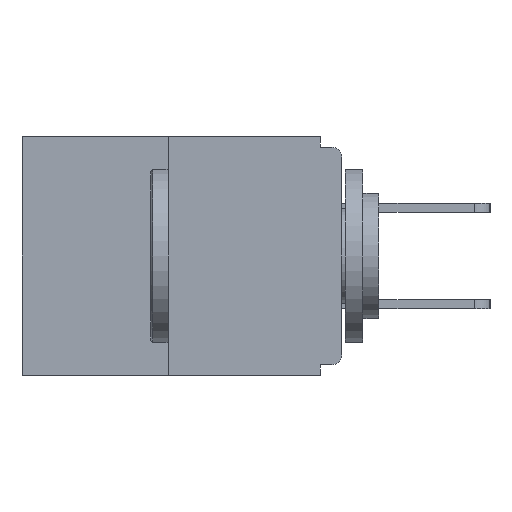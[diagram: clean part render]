
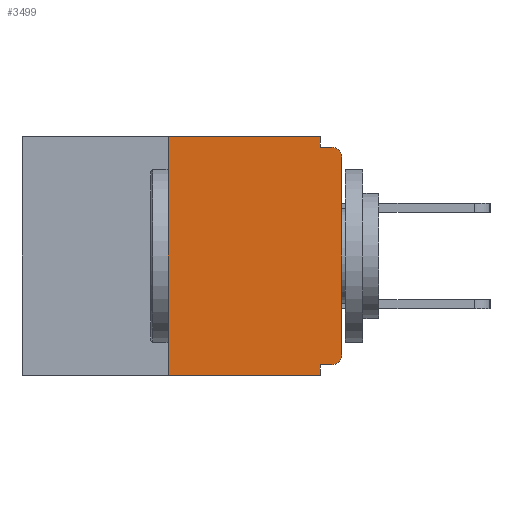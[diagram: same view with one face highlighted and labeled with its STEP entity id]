
A CAD part, left-side view. The second image highlights one B-rep face of the part: STEP entity #3499.
In plain terms, the highlighted planar face has unit normal (-1, 0, 0).
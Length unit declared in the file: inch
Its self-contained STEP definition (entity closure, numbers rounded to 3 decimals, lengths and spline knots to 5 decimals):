
#41 = CARTESIAN_POINT ( 'NONE',  ( 0., 0.015, -0.015 ) ) ;
#445 = CARTESIAN_POINT ( 'NONE',  ( 0., 0.015, -0.03 ) ) ;
#483 = DIRECTION ( 'NONE',  ( 1., 0., 0. ) ) ;
#566 = PLANE ( 'NONE',  #16511 ) ;
#655 = CARTESIAN_POINT ( 'NONE',  ( 0., 0.015, -0.328 ) ) ;
#1025 = CARTESIAN_POINT ( 'NONE',  ( 0., 0.031, 0. ) ) ;
#1550 = VERTEX_POINT ( 'NONE', #13295 ) ;
#2304 = VERTEX_POINT ( 'NONE', #9334 ) ;
#2338 = VERTEX_POINT ( 'NONE', #655 ) ;
#2637 = VERTEX_POINT ( 'NONE', #28172 ) ;
#2711 = DIRECTION ( 'NONE',  ( -1., 0., 0. ) ) ;
#2716 = DIRECTION ( 'NONE',  ( 0., -1., 0. ) ) ;
#3070 = VECTOR ( 'NONE', #3271, 39.37008 ) ;
#3271 = DIRECTION ( 'NONE',  ( 0., -1., 0. ) ) ;
#3492 = EDGE_CURVE ( 'NONE', #14573, #27161, #8986, .T. ) ;
#3499 = ADVANCED_FACE ( 'NONE', ( #24289 ), #566, .F. ) ;
#3878 = ORIENTED_EDGE ( 'NONE', *, *, #14083, .F. ) ;
#4466 = VERTEX_POINT ( 'NONE', #18391 ) ;
#4516 = VERTEX_POINT ( 'NONE', #1025 ) ;
#4928 = AXIS2_PLACEMENT_3D ( 'NONE', #20759, #5665, #27473 ) ;
#4995 = DIRECTION ( 'NONE',  ( 0., 0., -1. ) ) ;
#5268 = EDGE_CURVE ( 'NONE', #14573, #2637, #14663, .T. ) ;
#5332 = CARTESIAN_POINT ( 'NONE',  ( 0., 0.46, -0.343 ) ) ;
#5359 = EDGE_LOOP ( 'NONE', ( #6457, #19528, #24712, #18139, #14676, #10638, #19654, #18191, #3878, #10614 ) ) ;
#5665 = DIRECTION ( 'NONE',  ( -1., 0., 0. ) ) ;
#6179 = DIRECTION ( 'NONE',  ( 0., 0., -1. ) ) ;
#6457 = ORIENTED_EDGE ( 'NONE', *, *, #12551, .F. ) ;
#6842 = CARTESIAN_POINT ( 'NONE',  ( 0., 0.031, -0.015 ) ) ;
#6968 = CARTESIAN_POINT ( 'NONE',  ( 0., 0.46, 0. ) ) ;
#7500 = LINE ( 'NONE', #14070, #3070 ) ;
#8016 = VECTOR ( 'NONE', #6179, 39.37008 ) ;
#8986 = LINE ( 'NONE', #22368, #21553 ) ;
#9126 = CARTESIAN_POINT ( 'NONE',  ( 0., 0.25, 0. ) ) ;
#9263 = VERTEX_POINT ( 'NONE', #41 ) ;
#9334 = CARTESIAN_POINT ( 'NONE',  ( 0., 0., -0.313 ) ) ;
#9336 = DIRECTION ( 'NONE',  ( 0., 0., -1. ) ) ;
#9657 = EDGE_CURVE ( 'NONE', #4516, #13980, #14191, .T. ) ;
#9791 = VECTOR ( 'NONE', #2716, 39.37008 ) ;
#10184 = DIRECTION ( 'NONE',  ( 0., 0., -1. ) ) ;
#10614 = ORIENTED_EDGE ( 'NONE', *, *, #9657, .F. ) ;
#10638 = ORIENTED_EDGE ( 'NONE', *, *, #22454, .T. ) ;
#10742 = CARTESIAN_POINT ( 'NONE',  ( 0., 0.25, -0.343 ) ) ;
#12551 = EDGE_CURVE ( 'NONE', #27161, #4516, #7500, .T. ) ;
#13295 = CARTESIAN_POINT ( 'NONE',  ( 0., 0.031, -0.328 ) ) ;
#13980 = VERTEX_POINT ( 'NONE', #6842 ) ;
#14070 = CARTESIAN_POINT ( 'NONE',  ( 0., 0.46, 0. ) ) ;
#14083 = EDGE_CURVE ( 'NONE', #13980, #9263, #23731, .T. ) ;
#14116 = DIRECTION ( 'NONE',  ( 0., -1., 0. ) ) ;
#14143 = AXIS2_PLACEMENT_3D ( 'NONE', #445, #2711, #4995 ) ;
#14191 = LINE ( 'NONE', #14957, #8016 ) ;
#14364 = CARTESIAN_POINT ( 'NONE',  ( 0., 0., -0.328 ) ) ;
#14573 = VERTEX_POINT ( 'NONE', #10742 ) ;
#14663 = LINE ( 'NONE', #5332, #14994 ) ;
#14676 = ORIENTED_EDGE ( 'NONE', *, *, #25418, .F. ) ;
#14821 = VECTOR ( 'NONE', #19490, 39.37008 ) ;
#14957 = CARTESIAN_POINT ( 'NONE',  ( 0., 0.031, 0. ) ) ;
#14994 = VECTOR ( 'NONE', #14116, 39.37008 ) ;
#15132 = CIRCLE ( 'NONE', #4928, 0.015 ) ;
#15308 = EDGE_CURVE ( 'NONE', #4466, #9263, #28052, .T. ) ;
#15794 = VECTOR ( 'NONE', #10184, 39.37008 ) ;
#16511 = AXIS2_PLACEMENT_3D ( 'NONE', #6968, #483, #9336 ) ;
#17619 = CARTESIAN_POINT ( 'NONE',  ( 0., 0., 0. ) ) ;
#18021 = DIRECTION ( 'NONE',  ( 0., 0., 1. ) ) ;
#18139 = ORIENTED_EDGE ( 'NONE', *, *, #22733, .F. ) ;
#18191 = ORIENTED_EDGE ( 'NONE', *, *, #15308, .T. ) ;
#18300 = VECTOR ( 'NONE', #20893, 39.37008 ) ;
#18391 = CARTESIAN_POINT ( 'NONE',  ( 0., 0., -0.03 ) ) ;
#19306 = LINE ( 'NONE', #14364, #18300 ) ;
#19490 = DIRECTION ( 'NONE',  ( 0., 0., 1. ) ) ;
#19528 = ORIENTED_EDGE ( 'NONE', *, *, #3492, .F. ) ;
#19654 = ORIENTED_EDGE ( 'NONE', *, *, #21015, .T. ) ;
#19934 = LINE ( 'NONE', #17619, #14821 ) ;
#20759 = CARTESIAN_POINT ( 'NONE',  ( 0., 0.015, -0.313 ) ) ;
#20893 = DIRECTION ( 'NONE',  ( 0., 1., 0. ) ) ;
#21015 = EDGE_CURVE ( 'NONE', #2304, #4466, #19934, .T. ) ;
#21553 = VECTOR ( 'NONE', #18021, 39.37008 ) ;
#22368 = CARTESIAN_POINT ( 'NONE',  ( 0., 0.25, 0. ) ) ;
#22454 = EDGE_CURVE ( 'NONE', #2338, #2304, #15132, .T. ) ;
#22733 = EDGE_CURVE ( 'NONE', #1550, #2637, #27318, .T. ) ;
#22921 = CARTESIAN_POINT ( 'NONE',  ( 0., 0.031, -0.343 ) ) ;
#23731 = LINE ( 'NONE', #26873, #9791 ) ;
#24289 = FACE_OUTER_BOUND ( 'NONE', #5359, .T. ) ;
#24712 = ORIENTED_EDGE ( 'NONE', *, *, #5268, .T. ) ;
#25418 = EDGE_CURVE ( 'NONE', #2338, #1550, #19306, .T. ) ;
#26873 = CARTESIAN_POINT ( 'NONE',  ( 0., 0., -0.015 ) ) ;
#27161 = VERTEX_POINT ( 'NONE', #9126 ) ;
#27318 = LINE ( 'NONE', #22921, #15794 ) ;
#27473 = DIRECTION ( 'NONE',  ( 0., 0., -1. ) ) ;
#28052 = CIRCLE ( 'NONE', #14143, 0.015 ) ;
#28172 = CARTESIAN_POINT ( 'NONE',  ( 0., 0.031, -0.343 ) ) ;
